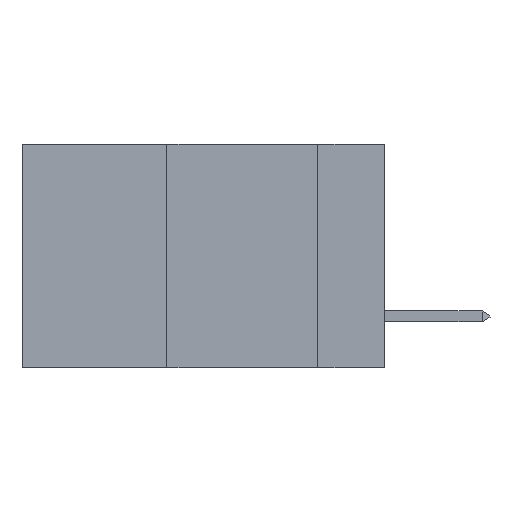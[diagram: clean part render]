
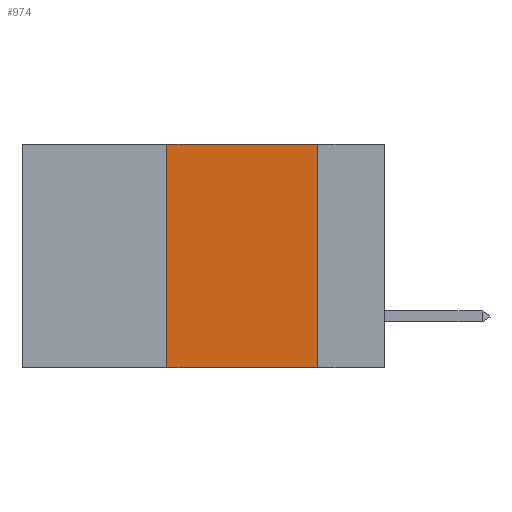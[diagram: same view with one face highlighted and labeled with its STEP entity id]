
A CAD part, left-side view. The second image highlights one B-rep face of the part: STEP entity #974.
In plain terms, the highlighted planar face has unit normal (-1, 0, 0).
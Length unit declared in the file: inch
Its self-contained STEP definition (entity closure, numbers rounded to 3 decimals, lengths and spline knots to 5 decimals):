
#441 = CARTESIAN_POINT ( 'NONE',  ( 0., 0.36, -0.37 ) ) ;
#974 = ADVANCED_FACE ( 'NONE', ( #8456 ), #2204, .F. ) ;
#1022 = LINE ( 'NONE', #6210, #4842 ) ;
#1172 = DIRECTION ( 'NONE',  ( 0., 0., -1. ) ) ;
#2114 = LINE ( 'NONE', #5507, #8177 ) ;
#2204 = PLANE ( 'NONE',  #7754 ) ;
#2354 = ORIENTED_EDGE ( 'NONE', *, *, #8539, .F. ) ;
#2740 = VERTEX_POINT ( 'NONE', #4403 ) ;
#2769 = VERTEX_POINT ( 'NONE', #441 ) ;
#3100 = DIRECTION ( 'NONE',  ( 1., 0., 0. ) ) ;
#3110 = DIRECTION ( 'NONE',  ( 0., 0., 1. ) ) ;
#3850 = CARTESIAN_POINT ( 'NONE',  ( 0., 0.6, 0. ) ) ;
#4137 = CARTESIAN_POINT ( 'NONE',  ( 0., 0.36, 0. ) ) ;
#4378 = EDGE_CURVE ( 'NONE', #9633, #2740, #8732, .T. ) ;
#4403 = CARTESIAN_POINT ( 'NONE',  ( 0., 0.11, 0. ) ) ;
#4581 = LINE ( 'NONE', #8690, #6535 ) ;
#4842 = VECTOR ( 'NONE', #7069, 39.37008 ) ;
#5507 = CARTESIAN_POINT ( 'NONE',  ( 0., 0.36, 0. ) ) ;
#6187 = ORIENTED_EDGE ( 'NONE', *, *, #8470, .F. ) ;
#6210 = CARTESIAN_POINT ( 'NONE',  ( 0., 0.6, -0.37 ) ) ;
#6535 = VECTOR ( 'NONE', #1172, 39.37008 ) ;
#6615 = VECTOR ( 'NONE', #10753, 39.37008 ) ;
#7069 = DIRECTION ( 'NONE',  ( 0., -1., 0. ) ) ;
#7339 = VERTEX_POINT ( 'NONE', #10785 ) ;
#7754 = AXIS2_PLACEMENT_3D ( 'NONE', #3850, #3100, #8750 ) ;
#8177 = VECTOR ( 'NONE', #3110, 39.37008 ) ;
#8345 = ORIENTED_EDGE ( 'NONE', *, *, #4378, .F. ) ;
#8456 = FACE_OUTER_BOUND ( 'NONE', #8921, .T. ) ;
#8470 = EDGE_CURVE ( 'NONE', #2740, #7339, #4581, .T. ) ;
#8539 = EDGE_CURVE ( 'NONE', #2769, #9633, #2114, .T. ) ;
#8690 = CARTESIAN_POINT ( 'NONE',  ( 0., 0.11, 0. ) ) ;
#8732 = LINE ( 'NONE', #10291, #6615 ) ;
#8750 = DIRECTION ( 'NONE',  ( 0., 0., -1. ) ) ;
#8921 = EDGE_LOOP ( 'NONE', ( #6187, #8345, #2354, #9102 ) ) ;
#9102 = ORIENTED_EDGE ( 'NONE', *, *, #9223, .T. ) ;
#9223 = EDGE_CURVE ( 'NONE', #2769, #7339, #1022, .T. ) ;
#9633 = VERTEX_POINT ( 'NONE', #4137 ) ;
#10291 = CARTESIAN_POINT ( 'NONE',  ( 0., 0.6, 0. ) ) ;
#10753 = DIRECTION ( 'NONE',  ( 0., -1., 0. ) ) ;
#10785 = CARTESIAN_POINT ( 'NONE',  ( 0., 0.11, -0.37 ) ) ;
